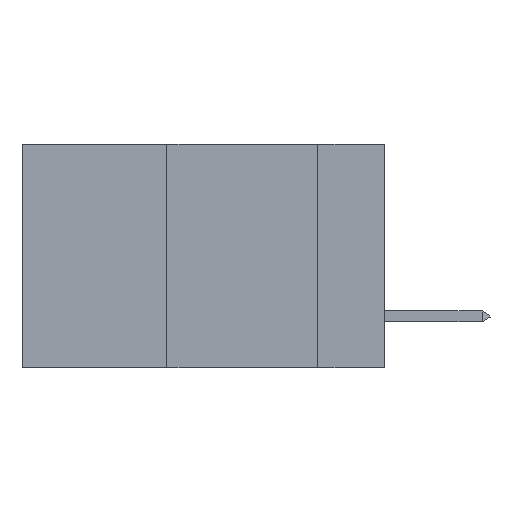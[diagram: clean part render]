
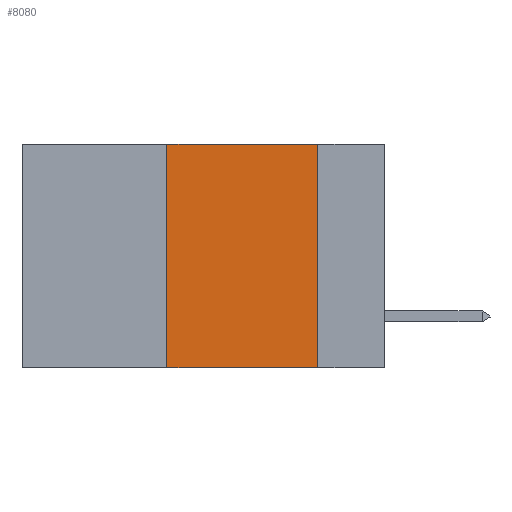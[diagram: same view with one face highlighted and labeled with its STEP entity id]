
A CAD part, left-side view. The second image highlights one B-rep face of the part: STEP entity #8080.
In plain terms, the highlighted planar face has unit normal (-1, 0, 0).
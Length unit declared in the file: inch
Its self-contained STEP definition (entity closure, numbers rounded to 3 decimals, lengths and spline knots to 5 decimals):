
#154 = EDGE_CURVE ( 'NONE', #39709, #15613, #23009, .T. ) ;
#1982 = DIRECTION ( 'NONE',  ( 1., 0., 0. ) ) ;
#2180 = ORIENTED_EDGE ( 'NONE', *, *, #40823, .F. ) ;
#2500 = VERTEX_POINT ( 'NONE', #32854 ) ;
#3424 = DIRECTION ( 'NONE',  ( 0., 0., -1. ) ) ;
#5578 = ORIENTED_EDGE ( 'NONE', *, *, #154, .T. ) ;
#6351 = VECTOR ( 'NONE', #3424, 39.37008 ) ;
#6761 = LINE ( 'NONE', #41885, #28424 ) ;
#7068 = EDGE_CURVE ( 'NONE', #24688, #2500, #16639, .T. ) ;
#7376 = VECTOR ( 'NONE', #47049, 39.37008 ) ;
#8080 = ADVANCED_FACE ( 'NONE', ( #35553 ), #21273, .F. ) ;
#9458 = ORIENTED_EDGE ( 'NONE', *, *, #7068, .F. ) ;
#11460 = DIRECTION ( 'NONE',  ( 0., 0., 1. ) ) ;
#11618 = CARTESIAN_POINT ( 'NONE',  ( 0., 0.36, 0. ) ) ;
#12961 = CARTESIAN_POINT ( 'NONE',  ( 0., 0.36, -0.37 ) ) ;
#15613 = VERTEX_POINT ( 'NONE', #48955 ) ;
#16639 = LINE ( 'NONE', #40127, #21434 ) ;
#16771 = DIRECTION ( 'NONE',  ( 0., -1., 0. ) ) ;
#19849 = CARTESIAN_POINT ( 'NONE',  ( 0., 0.6, -0.37 ) ) ;
#21273 = PLANE ( 'NONE',  #47718 ) ;
#21434 = VECTOR ( 'NONE', #16771, 39.37008 ) ;
#23009 = LINE ( 'NONE', #19849, #7376 ) ;
#24313 = CARTESIAN_POINT ( 'NONE',  ( 0., 0.6, 0. ) ) ;
#24688 = VERTEX_POINT ( 'NONE', #11618 ) ;
#24830 = DIRECTION ( 'NONE',  ( 0., 0., -1. ) ) ;
#28424 = VECTOR ( 'NONE', #11460, 39.37008 ) ;
#32854 = CARTESIAN_POINT ( 'NONE',  ( 0., 0.11, 0. ) ) ;
#33429 = LINE ( 'NONE', #34038, #6351 ) ;
#33466 = EDGE_CURVE ( 'NONE', #39709, #24688, #6761, .T. ) ;
#34038 = CARTESIAN_POINT ( 'NONE',  ( 0., 0.11, 0. ) ) ;
#35553 = FACE_OUTER_BOUND ( 'NONE', #43539, .T. ) ;
#39709 = VERTEX_POINT ( 'NONE', #12961 ) ;
#40127 = CARTESIAN_POINT ( 'NONE',  ( 0., 0.6, 0. ) ) ;
#40823 = EDGE_CURVE ( 'NONE', #2500, #15613, #33429, .T. ) ;
#41885 = CARTESIAN_POINT ( 'NONE',  ( 0., 0.36, 0. ) ) ;
#43539 = EDGE_LOOP ( 'NONE', ( #2180, #9458, #48504, #5578 ) ) ;
#47049 = DIRECTION ( 'NONE',  ( 0., -1., 0. ) ) ;
#47718 = AXIS2_PLACEMENT_3D ( 'NONE', #24313, #1982, #24830 ) ;
#48504 = ORIENTED_EDGE ( 'NONE', *, *, #33466, .F. ) ;
#48955 = CARTESIAN_POINT ( 'NONE',  ( 0., 0.11, -0.37 ) ) ;
